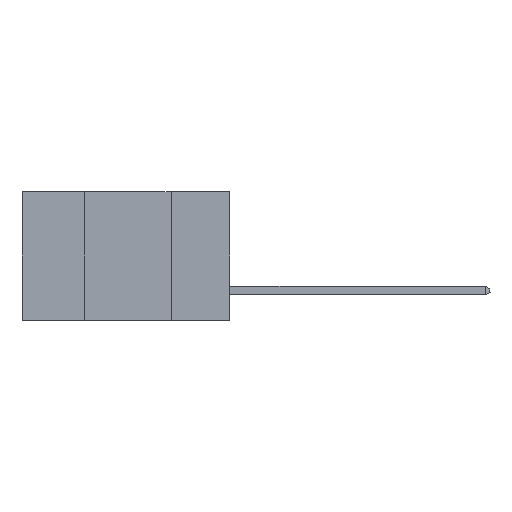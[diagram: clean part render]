
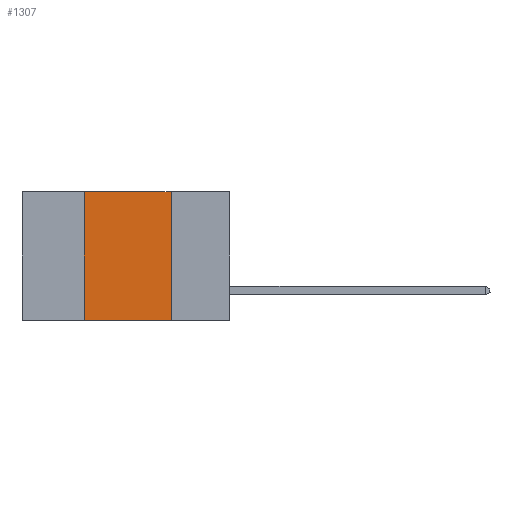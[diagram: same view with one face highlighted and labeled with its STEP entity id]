
A CAD part, left-side view. The second image highlights one B-rep face of the part: STEP entity #1307.
In plain terms, the highlighted planar face has unit normal (-1, 0, 0).
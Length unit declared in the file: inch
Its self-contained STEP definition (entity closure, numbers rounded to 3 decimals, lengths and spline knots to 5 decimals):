
#961 = DIRECTION ( 'NONE',  ( 0., 0., 1. ) ) ;
#1300 = VECTOR ( 'NONE', #6819, 39.37008 ) ;
#1307 = ADVANCED_FACE ( 'NONE', ( #7010 ), #11507, .F. ) ;
#1647 = EDGE_LOOP ( 'NONE', ( #2480, #2287, #7371, #11443 ) ) ;
#1981 = CARTESIAN_POINT ( 'NONE',  ( 0., 0.6, -0.37 ) ) ;
#2229 = CARTESIAN_POINT ( 'NONE',  ( 0., 0.17, 0. ) ) ;
#2287 = ORIENTED_EDGE ( 'NONE', *, *, #7693, .F. ) ;
#2467 = LINE ( 'NONE', #5947, #1300 ) ;
#2480 = ORIENTED_EDGE ( 'NONE', *, *, #5876, .F. ) ;
#2777 = AXIS2_PLACEMENT_3D ( 'NONE', #8838, #9720, #3242 ) ;
#3242 = DIRECTION ( 'NONE',  ( 0., 0., -1. ) ) ;
#4251 = CARTESIAN_POINT ( 'NONE',  ( 0., 0.17, 0. ) ) ;
#4546 = CARTESIAN_POINT ( 'NONE',  ( 0., 0.42, 0. ) ) ;
#4859 = VERTEX_POINT ( 'NONE', #4546 ) ;
#5688 = EDGE_CURVE ( 'NONE', #10283, #8725, #9082, .T. ) ;
#5876 = EDGE_CURVE ( 'NONE', #10878, #8725, #8782, .T. ) ;
#5947 = CARTESIAN_POINT ( 'NONE',  ( 0., 0.6, 0. ) ) ;
#6306 = VECTOR ( 'NONE', #9719, 39.37008 ) ;
#6819 = DIRECTION ( 'NONE',  ( 0., -1., 0. ) ) ;
#7010 = FACE_OUTER_BOUND ( 'NONE', #1647, .T. ) ;
#7371 = ORIENTED_EDGE ( 'NONE', *, *, #8778, .F. ) ;
#7590 = CARTESIAN_POINT ( 'NONE',  ( 0., 0.17, -0.37 ) ) ;
#7675 = CARTESIAN_POINT ( 'NONE',  ( 0., 0.42, 0. ) ) ;
#7693 = EDGE_CURVE ( 'NONE', #4859, #10878, #2467, .T. ) ;
#8633 = VECTOR ( 'NONE', #9361, 39.37008 ) ;
#8725 = VERTEX_POINT ( 'NONE', #7590 ) ;
#8778 = EDGE_CURVE ( 'NONE', #10283, #4859, #9165, .T. ) ;
#8782 = LINE ( 'NONE', #2229, #6306 ) ;
#8838 = CARTESIAN_POINT ( 'NONE',  ( 0., 0.6, 0. ) ) ;
#9082 = LINE ( 'NONE', #1981, #8633 ) ;
#9149 = CARTESIAN_POINT ( 'NONE',  ( 0., 0.42, -0.37 ) ) ;
#9165 = LINE ( 'NONE', #7675, #10927 ) ;
#9361 = DIRECTION ( 'NONE',  ( 0., -1., 0. ) ) ;
#9719 = DIRECTION ( 'NONE',  ( 0., 0., -1. ) ) ;
#9720 = DIRECTION ( 'NONE',  ( 1., 0., 0. ) ) ;
#10283 = VERTEX_POINT ( 'NONE', #9149 ) ;
#10878 = VERTEX_POINT ( 'NONE', #4251 ) ;
#10927 = VECTOR ( 'NONE', #961, 39.37008 ) ;
#11443 = ORIENTED_EDGE ( 'NONE', *, *, #5688, .T. ) ;
#11507 = PLANE ( 'NONE',  #2777 ) ;
